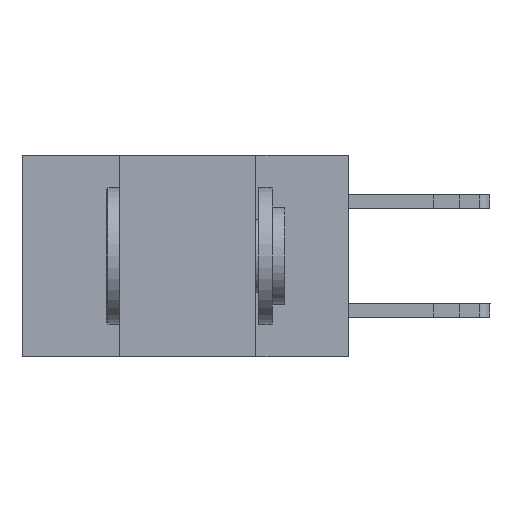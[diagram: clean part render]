
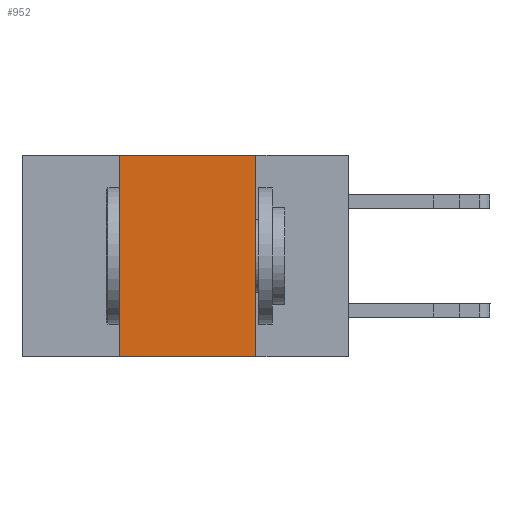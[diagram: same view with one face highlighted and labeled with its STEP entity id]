
A CAD part, left-side view. The second image highlights one B-rep face of the part: STEP entity #952.
In plain terms, the highlighted planar face has unit normal (-1, 0, 0).
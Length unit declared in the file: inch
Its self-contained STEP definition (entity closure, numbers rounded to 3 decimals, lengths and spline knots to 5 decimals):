
#310 = DIRECTION ( 'NONE',  ( 0., 0., -1. ) ) ;
#952 = ADVANCED_FACE ( 'NONE', ( #9057 ), #9166, .F. ) ;
#1494 = EDGE_CURVE ( 'NONE', #2756, #3753, #14830, .T. ) ;
#1669 = VECTOR ( 'NONE', #5318, 39.37008 ) ;
#2756 = VERTEX_POINT ( 'NONE', #14058 ) ;
#3390 = LINE ( 'NONE', #4394, #6307 ) ;
#3753 = VERTEX_POINT ( 'NONE', #13509 ) ;
#4337 = DIRECTION ( 'NONE',  ( 0., 0., 1. ) ) ;
#4394 = CARTESIAN_POINT ( 'NONE',  ( 0., 0.42, -0.37 ) ) ;
#4728 = EDGE_CURVE ( 'NONE', #2756, #8982, #3390, .T. ) ;
#4891 = LINE ( 'NONE', #5223, #1669 ) ;
#5131 = ORIENTED_EDGE ( 'NONE', *, *, #9042, .F. ) ;
#5223 = CARTESIAN_POINT ( 'NONE',  ( 0., 0.6, 0. ) ) ;
#5257 = EDGE_CURVE ( 'NONE', #10806, #3753, #12265, .T. ) ;
#5318 = DIRECTION ( 'NONE',  ( 0., -1., 0. ) ) ;
#5320 = ORIENTED_EDGE ( 'NONE', *, *, #5257, .F. ) ;
#6002 = CARTESIAN_POINT ( 'NONE',  ( 0., 0.42, 0. ) ) ;
#6307 = VECTOR ( 'NONE', #4337, 39.37008 ) ;
#6332 = ORIENTED_EDGE ( 'NONE', *, *, #1494, .T. ) ;
#7986 = DIRECTION ( 'NONE',  ( 0., 0., -1. ) ) ;
#8927 = VECTOR ( 'NONE', #7986, 39.37008 ) ;
#8982 = VERTEX_POINT ( 'NONE', #6002 ) ;
#9042 = EDGE_CURVE ( 'NONE', #8982, #10806, #4891, .T. ) ;
#9057 = FACE_OUTER_BOUND ( 'NONE', #14309, .T. ) ;
#9166 = PLANE ( 'NONE',  #12791 ) ;
#10806 = VERTEX_POINT ( 'NONE', #14251 ) ;
#10967 = DIRECTION ( 'NONE',  ( 1., 0., 0. ) ) ;
#11255 = VECTOR ( 'NONE', #12415, 39.37008 ) ;
#12265 = LINE ( 'NONE', #15104, #8927 ) ;
#12415 = DIRECTION ( 'NONE',  ( 0., -1., 0. ) ) ;
#12744 = CARTESIAN_POINT ( 'NONE',  ( 0., 0.6, 0. ) ) ;
#12791 = AXIS2_PLACEMENT_3D ( 'NONE', #12744, #10967, #310 ) ;
#13162 = CARTESIAN_POINT ( 'NONE',  ( 0., 0.6, -0.37 ) ) ;
#13509 = CARTESIAN_POINT ( 'NONE',  ( 0., 0.17, -0.37 ) ) ;
#14058 = CARTESIAN_POINT ( 'NONE',  ( 0., 0.42, -0.37 ) ) ;
#14251 = CARTESIAN_POINT ( 'NONE',  ( 0., 0.17, 0. ) ) ;
#14309 = EDGE_LOOP ( 'NONE', ( #5320, #5131, #15140, #6332 ) ) ;
#14830 = LINE ( 'NONE', #13162, #11255 ) ;
#15104 = CARTESIAN_POINT ( 'NONE',  ( 0., 0.17, -0.37 ) ) ;
#15140 = ORIENTED_EDGE ( 'NONE', *, *, #4728, .F. ) ;
